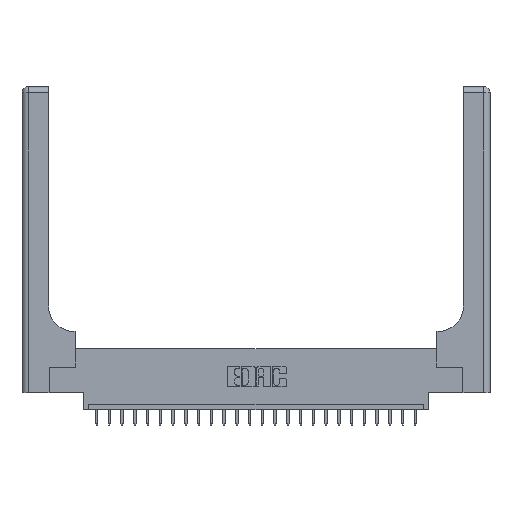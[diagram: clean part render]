
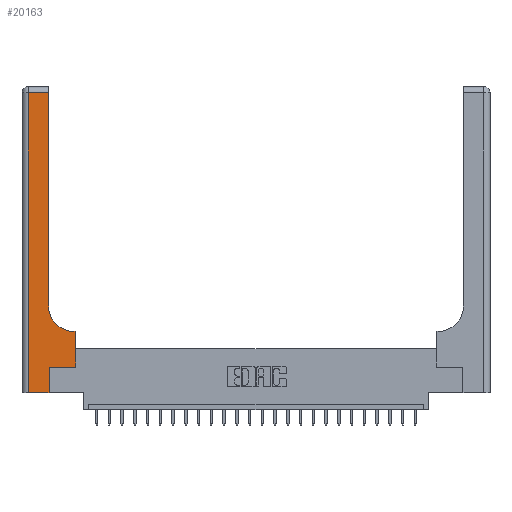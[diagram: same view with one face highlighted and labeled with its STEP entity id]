
A CAD part, top view. The second image highlights one B-rep face of the part: STEP entity #20163.
In plain terms, the highlighted planar face has unit normal (0, 0, 1).
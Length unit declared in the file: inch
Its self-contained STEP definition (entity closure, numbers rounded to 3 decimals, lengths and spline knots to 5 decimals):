
#173 = CARTESIAN_POINT ( 'NONE',  ( 0., 0., 0.37 ) ) ;
#362 = CARTESIAN_POINT ( 'NONE',  ( 0.265, 0., 0.37 ) ) ;
#363 = ORIENTED_EDGE ( 'NONE', *, *, #22925, .T. ) ;
#702 = ORIENTED_EDGE ( 'NONE', *, *, #22517, .T. ) ;
#910 = VECTOR ( 'NONE', #13286, 39.37008 ) ;
#1284 = CARTESIAN_POINT ( 'NONE',  ( 0., 3., 0.37 ) ) ;
#1773 = DIRECTION ( 'NONE',  ( 0., 0., -1. ) ) ;
#1785 = ORIENTED_EDGE ( 'NONE', *, *, #20362, .T. ) ;
#2005 = VERTEX_POINT ( 'NONE', #19695 ) ;
#2051 = EDGE_CURVE ( 'NONE', #5383, #14421, #6258, .T. ) ;
#2161 = DIRECTION ( 'NONE',  ( 0., -1., 0. ) ) ;
#2356 = AXIS2_PLACEMENT_3D ( 'NONE', #13858, #1773, #14787 ) ;
#2579 = DIRECTION ( 'NONE',  ( 1., 0., 0. ) ) ;
#3056 = EDGE_CURVE ( 'NONE', #23744, #22233, #18638, .T. ) ;
#3176 = CARTESIAN_POINT ( 'NONE',  ( 0.26, 2.94, 0.37 ) ) ;
#3950 = CARTESIAN_POINT ( 'NONE',  ( 0.51, 0.6, 0.37 ) ) ;
#4019 = ORIENTED_EDGE ( 'NONE', *, *, #6065, .T. ) ;
#4495 = DIRECTION ( 'NONE',  ( 0., 1., 0. ) ) ;
#4779 = CARTESIAN_POINT ( 'NONE',  ( 0.26, 0.6, 0.37 ) ) ;
#5383 = VERTEX_POINT ( 'NONE', #3950 ) ;
#5978 = ORIENTED_EDGE ( 'NONE', *, *, #6013, .T. ) ;
#6013 = EDGE_CURVE ( 'NONE', #10438, #5383, #14141, .T. ) ;
#6065 = EDGE_CURVE ( 'NONE', #22233, #10699, #9610, .T. ) ;
#6258 = CIRCLE ( 'NONE', #2356, 0.25 ) ;
#6743 = VECTOR ( 'NONE', #22652, 39.37008 ) ;
#6844 = DIRECTION ( 'NONE',  ( -1., 0., 0. ) ) ;
#6894 = FACE_OUTER_BOUND ( 'NONE', #19009, .T. ) ;
#6973 = ORIENTED_EDGE ( 'NONE', *, *, #20885, .T. ) ;
#7034 = EDGE_CURVE ( 'NONE', #8846, #2005, #22799, .T. ) ;
#8289 = VECTOR ( 'NONE', #20268, 39.37008 ) ;
#8583 = ORIENTED_EDGE ( 'NONE', *, *, #2051, .T. ) ;
#8723 = DIRECTION ( 'NONE',  ( -1., 0., 0. ) ) ;
#8846 = VERTEX_POINT ( 'NONE', #9305 ) ;
#9122 = CARTESIAN_POINT ( 'NONE',  ( 0.528, 0.25, 0.37 ) ) ;
#9305 = CARTESIAN_POINT ( 'NONE',  ( 0.265, 0.25, 0.37 ) ) ;
#9610 = LINE ( 'NONE', #16761, #11906 ) ;
#10095 = LINE ( 'NONE', #362, #11454 ) ;
#10438 = VERTEX_POINT ( 'NONE', #18403 ) ;
#10699 = VERTEX_POINT ( 'NONE', #21333 ) ;
#10885 = DIRECTION ( 'NONE',  ( 0., 0., -1. ) ) ;
#11454 = VECTOR ( 'NONE', #4495, 39.37008 ) ;
#11530 = VECTOR ( 'NONE', #6844, 39.37008 ) ;
#11906 = VECTOR ( 'NONE', #2161, 39.37008 ) ;
#12761 = ORIENTED_EDGE ( 'NONE', *, *, #3056, .T. ) ;
#13286 = DIRECTION ( 'NONE',  ( 0., 1., 0. ) ) ;
#13776 = LINE ( 'NONE', #17412, #910 ) ;
#13858 = CARTESIAN_POINT ( 'NONE',  ( 0.51, 0.85, 0.37 ) ) ;
#14141 = LINE ( 'NONE', #4779, #11530 ) ;
#14284 = ORIENTED_EDGE ( 'NONE', *, *, #7034, .T. ) ;
#14421 = VERTEX_POINT ( 'NONE', #14493 ) ;
#14493 = CARTESIAN_POINT ( 'NONE',  ( 0.26, 0.85, 0.37 ) ) ;
#14787 = DIRECTION ( 'NONE',  ( 1., 0., 0. ) ) ;
#16646 = DIRECTION ( 'NONE',  ( 0., 1., 0. ) ) ;
#16761 = CARTESIAN_POINT ( 'NONE',  ( 0.06, 3., 0.37 ) ) ;
#17412 = CARTESIAN_POINT ( 'NONE',  ( 0.26, 3., 0.37 ) ) ;
#17659 = CARTESIAN_POINT ( 'NONE',  ( 0.06, 2.94, 0.37 ) ) ;
#18403 = CARTESIAN_POINT ( 'NONE',  ( 0.528, 0.6, 0.37 ) ) ;
#18638 = LINE ( 'NONE', #20353, #6743 ) ;
#18674 = LINE ( 'NONE', #173, #8289 ) ;
#19009 = EDGE_LOOP ( 'NONE', ( #6973, #12761, #4019, #1785, #702, #14284, #363, #5978, #8583 ) ) ;
#19171 = CARTESIAN_POINT ( 'NONE',  ( 0.265, 0., 0.37 ) ) ;
#19638 = VECTOR ( 'NONE', #16646, 39.37008 ) ;
#19670 = PLANE ( 'NONE',  #22278 ) ;
#19695 = CARTESIAN_POINT ( 'NONE',  ( 0.528, 0.25, 0.37 ) ) ;
#20163 = ADVANCED_FACE ( 'NONE', ( #6894 ), #19670, .F. ) ;
#20268 = DIRECTION ( 'NONE',  ( 1., 0., 0. ) ) ;
#20353 = CARTESIAN_POINT ( 'NONE',  ( 0., 2.94, 0.37 ) ) ;
#20362 = EDGE_CURVE ( 'NONE', #10699, #23174, #18674, .T. ) ;
#20885 = EDGE_CURVE ( 'NONE', #14421, #23744, #13776, .T. ) ;
#21333 = CARTESIAN_POINT ( 'NONE',  ( 0.06, 0., 0.37 ) ) ;
#22137 = LINE ( 'NONE', #9122, #19638 ) ;
#22233 = VERTEX_POINT ( 'NONE', #17659 ) ;
#22278 = AXIS2_PLACEMENT_3D ( 'NONE', #1284, #10885, #8723 ) ;
#22517 = EDGE_CURVE ( 'NONE', #23174, #8846, #10095, .T. ) ;
#22652 = DIRECTION ( 'NONE',  ( -1., 0., 0. ) ) ;
#22674 = CARTESIAN_POINT ( 'NONE',  ( 0.265, 0.25, 0.37 ) ) ;
#22799 = LINE ( 'NONE', #22674, #23188 ) ;
#22925 = EDGE_CURVE ( 'NONE', #2005, #10438, #22137, .T. ) ;
#23174 = VERTEX_POINT ( 'NONE', #19171 ) ;
#23188 = VECTOR ( 'NONE', #2579, 39.37008 ) ;
#23744 = VERTEX_POINT ( 'NONE', #3176 ) ;
